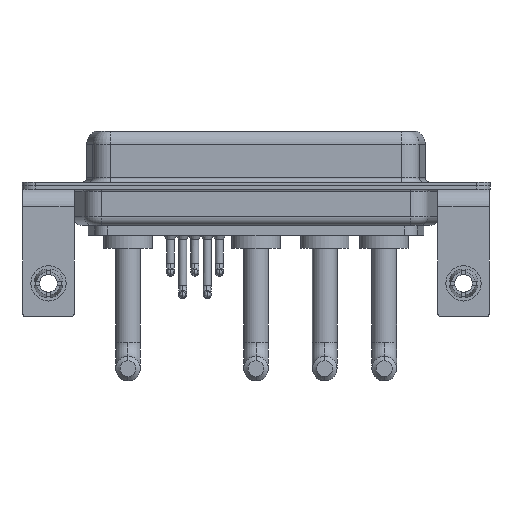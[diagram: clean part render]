
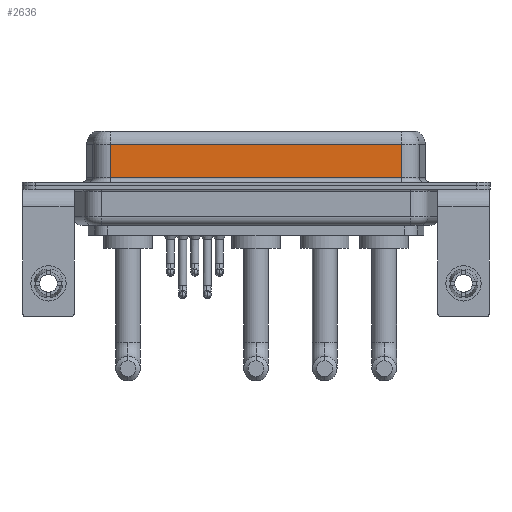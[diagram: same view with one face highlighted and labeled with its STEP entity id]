
A CAD part, front view. The second image highlights one B-rep face of the part: STEP entity #2636.
In plain terms, the highlighted planar face has unit normal (0, -1, 0).
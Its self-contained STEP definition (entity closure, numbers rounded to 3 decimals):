
#323 = CARTESIAN_POINT ( 'NONE',  ( 7.013, -3.95, 6.4 ) ) ;
#397 = LINE ( 'NONE', #16810, #6771 ) ;
#694 = EDGE_CURVE ( 'NONE', #15876, #5660, #3075, .T. ) ;
#1037 = CARTESIAN_POINT ( 'NONE',  ( 40.037, -3.95, 6.4 ) ) ;
#1361 = ORIENTED_EDGE ( 'NONE', *, *, #9381, .T. ) ;
#1561 = CARTESIAN_POINT ( 'NONE',  ( 40.037, -3.95, 4.65 ) ) ;
#2385 = LINE ( 'NONE', #8549, #6872 ) ;
#2632 = CARTESIAN_POINT ( 'NONE',  ( 7.013, -3.95, 4.65 ) ) ;
#2636 = ADVANCED_FACE ( 'NONE', ( #4120 ), #14772, .F. ) ;
#3075 = LINE ( 'NONE', #15817, #12661 ) ;
#3177 = DIRECTION ( 'NONE',  ( -1., 0., 0. ) ) ;
#3449 = CARTESIAN_POINT ( 'NONE',  ( 40.037, -3.95, 0.9 ) ) ;
#4120 = FACE_OUTER_BOUND ( 'NONE', #19510, .T. ) ;
#4774 = ORIENTED_EDGE ( 'NONE', *, *, #15602, .T. ) ;
#4867 = ORIENTED_EDGE ( 'NONE', *, *, #694, .T. ) ;
#5642 = VERTEX_POINT ( 'NONE', #1561 ) ;
#5660 = VERTEX_POINT ( 'NONE', #3449 ) ;
#5916 = VERTEX_POINT ( 'NONE', #2632 ) ;
#6771 = VECTOR ( 'NONE', #3177, 1000. ) ;
#6872 = VECTOR ( 'NONE', #19075, 1000. ) ;
#6910 = DIRECTION ( 'NONE',  ( 0., 1., 0. ) ) ;
#8242 = VECTOR ( 'NONE', #18119, 1000. ) ;
#8364 = CARTESIAN_POINT ( 'NONE',  ( 7.013, -3.95, 0.9 ) ) ;
#8549 = CARTESIAN_POINT ( 'NONE',  ( 40.037, -3.95, 6.4 ) ) ;
#9381 = EDGE_CURVE ( 'NONE', #5642, #5916, #397, .T. ) ;
#10206 = AXIS2_PLACEMENT_3D ( 'NONE', #1037, #6910, #12623 ) ;
#12623 = DIRECTION ( 'NONE',  ( 0., 0., 1. ) ) ;
#12639 = EDGE_CURVE ( 'NONE', #5642, #5660, #2385, .T. ) ;
#12661 = VECTOR ( 'NONE', #14220, 1000. ) ;
#13783 = ORIENTED_EDGE ( 'NONE', *, *, #12639, .F. ) ;
#14220 = DIRECTION ( 'NONE',  ( 1., 0., 0. ) ) ;
#14772 = PLANE ( 'NONE',  #10206 ) ;
#15162 = LINE ( 'NONE', #323, #8242 ) ;
#15602 = EDGE_CURVE ( 'NONE', #5916, #15876, #15162, .T. ) ;
#15817 = CARTESIAN_POINT ( 'NONE',  ( 40.037, -3.95, 0.9 ) ) ;
#15876 = VERTEX_POINT ( 'NONE', #8364 ) ;
#16810 = CARTESIAN_POINT ( 'NONE',  ( 40.037, -3.95, 4.65 ) ) ;
#18119 = DIRECTION ( 'NONE',  ( 0., 0., -1. ) ) ;
#19075 = DIRECTION ( 'NONE',  ( 0., 0., -1. ) ) ;
#19510 = EDGE_LOOP ( 'NONE', ( #13783, #1361, #4774, #4867 ) ) ;
